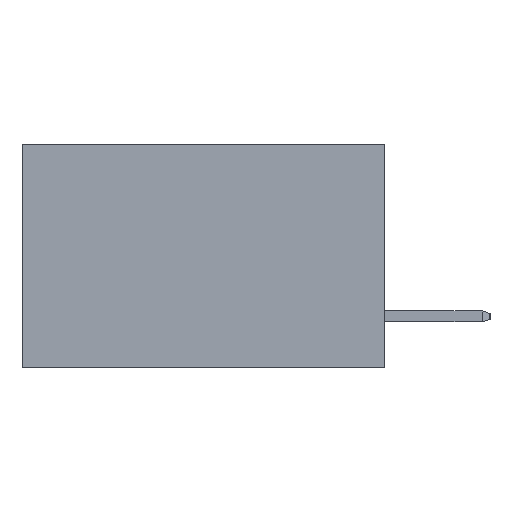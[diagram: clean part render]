
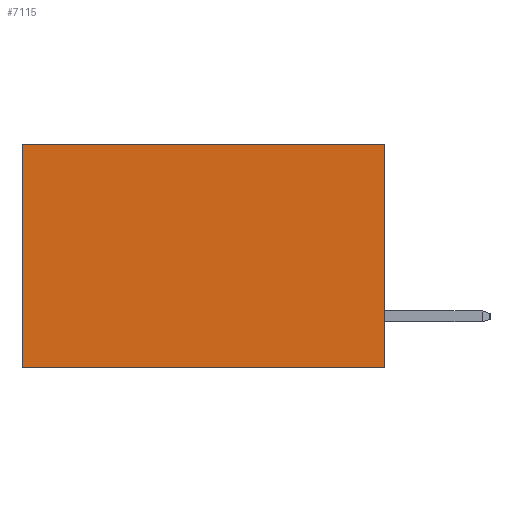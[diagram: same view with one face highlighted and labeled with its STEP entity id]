
A CAD part, left-side view. The second image highlights one B-rep face of the part: STEP entity #7115.
In plain terms, the highlighted planar face has unit normal (-1, 0, 0).
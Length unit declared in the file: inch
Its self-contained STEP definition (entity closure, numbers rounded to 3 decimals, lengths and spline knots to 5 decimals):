
#492 = CARTESIAN_POINT ( 'NONE',  ( 0.298, 0.6, 0. ) ) ;
#1416 = VERTEX_POINT ( 'NONE', #1751 ) ;
#1751 = CARTESIAN_POINT ( 'NONE',  ( 0.298, 0.6, -0.37 ) ) ;
#4676 = EDGE_CURVE ( 'NONE', #18463, #7311, #5770, .T. ) ;
#5289 = EDGE_CURVE ( 'NONE', #18526, #1416, #23352, .T. ) ;
#5770 = LINE ( 'NONE', #12780, #18297 ) ;
#5865 = DIRECTION ( 'NONE',  ( 0., 0., -1. ) ) ;
#5992 = VECTOR ( 'NONE', #19391, 39.37008 ) ;
#7115 = ADVANCED_FACE ( 'NONE', ( #15905 ), #21761, .F. ) ;
#7311 = VERTEX_POINT ( 'NONE', #27174 ) ;
#10108 = DIRECTION ( 'NONE',  ( 1., 0., 0. ) ) ;
#10897 = ORIENTED_EDGE ( 'NONE', *, *, #4676, .T. ) ;
#12257 = LINE ( 'NONE', #492, #5992 ) ;
#12631 = DIRECTION ( 'NONE',  ( 0., 1., 0. ) ) ;
#12780 = CARTESIAN_POINT ( 'NONE',  ( 0.298, 0., 0. ) ) ;
#13362 = VECTOR ( 'NONE', #5865, 39.37008 ) ;
#13688 = LINE ( 'NONE', #15271, #13362 ) ;
#15063 = DIRECTION ( 'NONE',  ( 0., 1., 0. ) ) ;
#15271 = CARTESIAN_POINT ( 'NONE',  ( 0.298, 0., 0. ) ) ;
#15905 = FACE_OUTER_BOUND ( 'NONE', #26428, .T. ) ;
#17156 = VECTOR ( 'NONE', #12631, 39.37008 ) ;
#18297 = VECTOR ( 'NONE', #15063, 39.37008 ) ;
#18463 = VERTEX_POINT ( 'NONE', #24738 ) ;
#18526 = VERTEX_POINT ( 'NONE', #21414 ) ;
#19391 = DIRECTION ( 'NONE',  ( 0., 0., -1. ) ) ;
#19631 = CARTESIAN_POINT ( 'NONE',  ( 0.298, 0., -0.37 ) ) ;
#20002 = ORIENTED_EDGE ( 'NONE', *, *, #20873, .F. ) ;
#20044 = EDGE_CURVE ( 'NONE', #7311, #1416, #12257, .T. ) ;
#20850 = ORIENTED_EDGE ( 'NONE', *, *, #5289, .F. ) ;
#20873 = EDGE_CURVE ( 'NONE', #18463, #18526, #13688, .T. ) ;
#21414 = CARTESIAN_POINT ( 'NONE',  ( 0.298, 0., -0.37 ) ) ;
#21761 = PLANE ( 'NONE',  #28767 ) ;
#23352 = LINE ( 'NONE', #19631, #17156 ) ;
#24127 = CARTESIAN_POINT ( 'NONE',  ( 0.298, 0., 0. ) ) ;
#24738 = CARTESIAN_POINT ( 'NONE',  ( 0.298, 0., 0. ) ) ;
#25698 = ORIENTED_EDGE ( 'NONE', *, *, #20044, .T. ) ;
#26428 = EDGE_LOOP ( 'NONE', ( #25698, #20850, #20002, #10897 ) ) ;
#26476 = DIRECTION ( 'NONE',  ( 0., 0., -1. ) ) ;
#27174 = CARTESIAN_POINT ( 'NONE',  ( 0.298, 0.6, 0. ) ) ;
#28767 = AXIS2_PLACEMENT_3D ( 'NONE', #24127, #10108, #26476 ) ;
